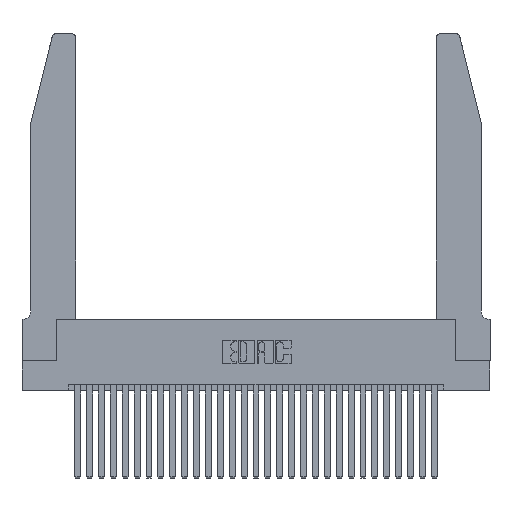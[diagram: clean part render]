
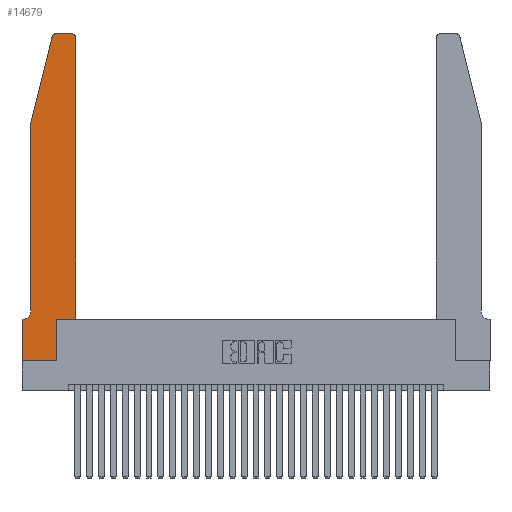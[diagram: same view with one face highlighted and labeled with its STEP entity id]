
A CAD part, top view. The second image highlights one B-rep face of the part: STEP entity #14679.
In plain terms, the highlighted planar face has unit normal (0, 0, 1).
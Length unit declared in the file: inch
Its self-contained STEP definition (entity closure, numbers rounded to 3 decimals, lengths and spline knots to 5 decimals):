
#418 = LINE ( 'NONE', #25442, #24624 ) ;
#552 = VECTOR ( 'NONE', #6811, 39.37008 ) ;
#963 = VERTEX_POINT ( 'NONE', #6507 ) ;
#1051 = EDGE_CURVE ( 'NONE', #26029, #1960, #15982, .T. ) ;
#1084 = DIRECTION ( 'NONE',  ( 1., 0., 0. ) ) ;
#1399 = EDGE_LOOP ( 'NONE', ( #8782, #19560, #9642, #27353, #13389, #15213, #22246, #16870, #8599, #26809, #6084, #13223 ) ) ;
#1864 = CARTESIAN_POINT ( 'NONE',  ( 0.0755, 2., 0.37 ) ) ;
#1960 = VERTEX_POINT ( 'NONE', #26092 ) ;
#2287 = EDGE_CURVE ( 'NONE', #23206, #22974, #24677, .T. ) ;
#2663 = VECTOR ( 'NONE', #15854, 39.37008 ) ;
#2941 = EDGE_CURVE ( 'NONE', #963, #4568, #8795, .T. ) ;
#3356 = VECTOR ( 'NONE', #10000, 39.37008 ) ;
#3378 = FACE_OUTER_BOUND ( 'NONE', #1399, .T. ) ;
#3464 = AXIS2_PLACEMENT_3D ( 'NONE', #12695, #17610, #1084 ) ;
#4360 = DIRECTION ( 'NONE',  ( -1., 0., 0. ) ) ;
#4417 = CARTESIAN_POINT ( 'NONE',  ( 0.4205, 2.72, 0.37 ) ) ;
#4474 = CARTESIAN_POINT ( 'NONE',  ( 0.2865, 0.35, 0.37 ) ) ;
#4568 = VERTEX_POINT ( 'NONE', #27083 ) ;
#6084 = ORIENTED_EDGE ( 'NONE', *, *, #11720, .T. ) ;
#6146 = AXIS2_PLACEMENT_3D ( 'NONE', #24119, #7701, #12446 ) ;
#6417 = CARTESIAN_POINT ( 'NONE',  ( 0.0755, 2., 0.37 ) ) ;
#6451 = CARTESIAN_POINT ( 'NONE',  ( 0., 0., 0.37 ) ) ;
#6507 = CARTESIAN_POINT ( 'NONE',  ( 0.4205, 2.75, 0.37 ) ) ;
#6531 = LINE ( 'NONE', #6451, #29653 ) ;
#6811 = DIRECTION ( 'NONE',  ( -1., 0., 0. ) ) ;
#6860 = CARTESIAN_POINT ( 'NONE',  ( 0., 0., 0.37 ) ) ;
#7011 = CARTESIAN_POINT ( 'NONE',  ( 0.0755, 0.35, 0.37 ) ) ;
#7701 = DIRECTION ( 'NONE',  ( 0., 0., 1. ) ) ;
#7878 = VERTEX_POINT ( 'NONE', #30296 ) ;
#7908 = CIRCLE ( 'NONE', #6146, 0.03 ) ;
#7933 = PLANE ( 'NONE',  #3464 ) ;
#8240 = DIRECTION ( 'NONE',  ( 0., 1., 0. ) ) ;
#8599 = ORIENTED_EDGE ( 'NONE', *, *, #2287, .T. ) ;
#8688 = EDGE_CURVE ( 'NONE', #22974, #23419, #418, .T. ) ;
#8782 = ORIENTED_EDGE ( 'NONE', *, *, #2941, .T. ) ;
#8795 = LINE ( 'NONE', #25005, #15803 ) ;
#8824 = DIRECTION ( 'NONE',  ( 1., 0., 0. ) ) ;
#9284 = CARTESIAN_POINT ( 'NONE',  ( 0.0055, 0.42, 0.37 ) ) ;
#9382 = EDGE_CURVE ( 'NONE', #15825, #26029, #21269, .T. ) ;
#9642 = ORIENTED_EDGE ( 'NONE', *, *, #24859, .T. ) ;
#10000 = DIRECTION ( 'NONE',  ( -0.239, -0.971, 0. ) ) ;
#10986 = EDGE_CURVE ( 'NONE', #19965, #963, #15341, .T. ) ;
#11644 = DIRECTION ( 'NONE',  ( 0., -1., 0. ) ) ;
#11672 = DIRECTION ( 'NONE',  ( 1., 0., 0. ) ) ;
#11720 = EDGE_CURVE ( 'NONE', #23419, #19965, #12342, .T. ) ;
#12021 = VERTEX_POINT ( 'NONE', #1864 ) ;
#12342 = LINE ( 'NONE', #29583, #17471 ) ;
#12446 = DIRECTION ( 'NONE',  ( 1., 0., 0. ) ) ;
#12695 = CARTESIAN_POINT ( 'NONE',  ( 0., 0.35, 0.37 ) ) ;
#13223 = ORIENTED_EDGE ( 'NONE', *, *, #10986, .T. ) ;
#13389 = ORIENTED_EDGE ( 'NONE', *, *, #9382, .T. ) ;
#13473 = VECTOR ( 'NONE', #11644, 39.37008 ) ;
#13681 = DIRECTION ( 'NONE',  ( 0., 0., 1. ) ) ;
#14679 = ADVANCED_FACE ( 'NONE', ( #3378 ), #7933, .T. ) ;
#15213 = ORIENTED_EDGE ( 'NONE', *, *, #1051, .T. ) ;
#15341 = CIRCLE ( 'NONE', #18540, 0.03 ) ;
#15803 = VECTOR ( 'NONE', #27955, 39.37008 ) ;
#15825 = VERTEX_POINT ( 'NONE', #19412 ) ;
#15854 = DIRECTION ( 'NONE',  ( 0., 1., 0. ) ) ;
#15982 = LINE ( 'NONE', #7011, #552 ) ;
#16178 = CARTESIAN_POINT ( 'NONE',  ( 0.4505, 2.72, 0.37 ) ) ;
#16466 = CARTESIAN_POINT ( 'NONE',  ( 0.0055, 0.35, 0.37 ) ) ;
#16788 = VERTEX_POINT ( 'NONE', #17995 ) ;
#16870 = ORIENTED_EDGE ( 'NONE', *, *, #27039, .T. ) ;
#17471 = VECTOR ( 'NONE', #8240, 39.37008 ) ;
#17610 = DIRECTION ( 'NONE',  ( 0., 0., 1. ) ) ;
#17995 = CARTESIAN_POINT ( 'NONE',  ( 0.25487, 2.72718, 0.37 ) ) ;
#18263 = VECTOR ( 'NONE', #23292, 39.37008 ) ;
#18540 = AXIS2_PLACEMENT_3D ( 'NONE', #4417, #13681, #20835 ) ;
#19412 = CARTESIAN_POINT ( 'NONE',  ( 0.0755, 0.42, 0.37 ) ) ;
#19560 = ORIENTED_EDGE ( 'NONE', *, *, #21839, .T. ) ;
#19965 = VERTEX_POINT ( 'NONE', #16178 ) ;
#20477 = CARTESIAN_POINT ( 'NONE',  ( 0.2865, 0., 0.37 ) ) ;
#20835 = DIRECTION ( 'NONE',  ( 1., 0., 0. ) ) ;
#21269 = CIRCLE ( 'NONE', #24998, 0.07 ) ;
#21839 = EDGE_CURVE ( 'NONE', #4568, #16788, #7908, .T. ) ;
#22074 = LINE ( 'NONE', #26347, #3356 ) ;
#22246 = ORIENTED_EDGE ( 'NONE', *, *, #27140, .T. ) ;
#22974 = VERTEX_POINT ( 'NONE', #4474 ) ;
#23206 = VERTEX_POINT ( 'NONE', #20477 ) ;
#23292 = DIRECTION ( 'NONE',  ( 0., -1., 0. ) ) ;
#23379 = LINE ( 'NONE', #6417, #13473 ) ;
#23419 = VERTEX_POINT ( 'NONE', #27640 ) ;
#24119 = CARTESIAN_POINT ( 'NONE',  ( 0.284, 2.72, 0.37 ) ) ;
#24624 = VECTOR ( 'NONE', #11672, 39.37008 ) ;
#24677 = LINE ( 'NONE', #27206, #2663 ) ;
#24859 = EDGE_CURVE ( 'NONE', #16788, #12021, #22074, .T. ) ;
#24998 = AXIS2_PLACEMENT_3D ( 'NONE', #9284, #25794, #4360 ) ;
#25005 = CARTESIAN_POINT ( 'NONE',  ( 0.2605, 2.75, 0.37 ) ) ;
#25442 = CARTESIAN_POINT ( 'NONE',  ( 0.4505, 0.35, 0.37 ) ) ;
#25794 = DIRECTION ( 'NONE',  ( 0., 0., -1. ) ) ;
#26029 = VERTEX_POINT ( 'NONE', #16466 ) ;
#26092 = CARTESIAN_POINT ( 'NONE',  ( 0., 0.35, 0.37 ) ) ;
#26347 = CARTESIAN_POINT ( 'NONE',  ( 0.0755, 2., 0.37 ) ) ;
#26809 = ORIENTED_EDGE ( 'NONE', *, *, #8688, .T. ) ;
#27039 = EDGE_CURVE ( 'NONE', #7878, #23206, #6531, .T. ) ;
#27083 = CARTESIAN_POINT ( 'NONE',  ( 0.284, 2.75, 0.37 ) ) ;
#27140 = EDGE_CURVE ( 'NONE', #1960, #7878, #27788, .T. ) ;
#27206 = CARTESIAN_POINT ( 'NONE',  ( 0.2865, 0.35, 0.37 ) ) ;
#27353 = ORIENTED_EDGE ( 'NONE', *, *, #27784, .T. ) ;
#27640 = CARTESIAN_POINT ( 'NONE',  ( 0.4505, 0.35, 0.37 ) ) ;
#27784 = EDGE_CURVE ( 'NONE', #12021, #15825, #23379, .T. ) ;
#27788 = LINE ( 'NONE', #6860, #18263 ) ;
#27955 = DIRECTION ( 'NONE',  ( -1., 0., 0. ) ) ;
#29583 = CARTESIAN_POINT ( 'NONE',  ( 0.4505, 0.35, 0.37 ) ) ;
#29653 = VECTOR ( 'NONE', #8824, 39.37008 ) ;
#30296 = CARTESIAN_POINT ( 'NONE',  ( 0., 0., 0.37 ) ) ;
